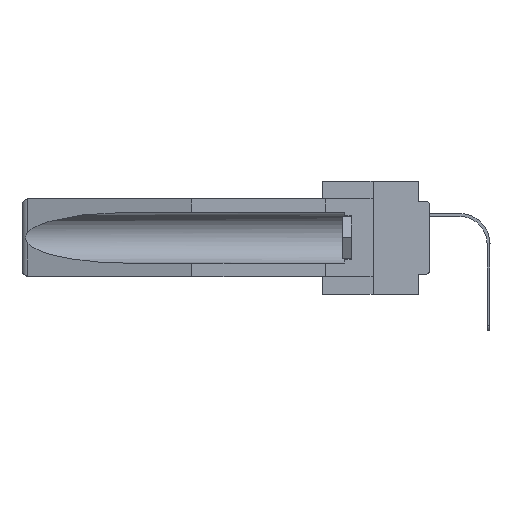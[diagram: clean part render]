
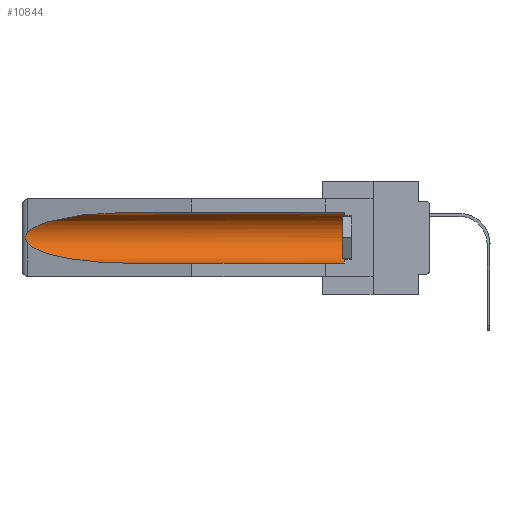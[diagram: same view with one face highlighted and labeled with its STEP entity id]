
A CAD part, left-side view. The second image highlights one B-rep face of the part: STEP entity #10844.
In plain terms, the highlighted cylindrical face has radius 2.857 mm (diameter 5.715 mm), a partial arc.
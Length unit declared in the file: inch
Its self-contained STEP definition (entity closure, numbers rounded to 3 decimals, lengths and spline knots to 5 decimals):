
#101 = CARTESIAN_POINT ( 'NONE',  ( 0.155, 1.07973, -0.059 ) ) ;
#251 = EDGE_CURVE ( 'NONE', #33269, #22558, #8034, .T. ) ;
#351 = ORIENTED_EDGE ( 'NONE', *, *, #16936, .T. ) ;
#2207 = CARTESIAN_POINT ( 'NONE',  ( 0.26537, 1.52718, -0.19328 ) ) ;
#2645 = FACE_OUTER_BOUND ( 'NONE', #35296, .T. ) ;
#2699 = CARTESIAN_POINT ( 'NONE',  ( 0.21114, 1.30732, -0.059 ) ) ;
#2713 = CARTESIAN_POINT ( 'NONE',  ( 0.26537, 1.52718, -0.14972 ) ) ;
#4264 = VERTEX_POINT ( 'NONE', #10974 ) ;
#4748 = CARTESIAN_POINT ( 'NONE',  ( 0.2675, 1.53308, -0.17534 ) ) ;
#4866 = DIRECTION ( 'NONE',  ( 0., 1., 0. ) ) ;
#5218 = CARTESIAN_POINT ( 'NONE',  ( 0.155, -0.30754, -0.1715 ) ) ;
#6916 =( BOUNDED_CURVE ( )  B_SPLINE_CURVE ( 3, ( #28275, #2699, #36361, #19280 ),
 .UNSPECIFIED., .F., .F. ) 
 B_SPLINE_CURVE_WITH_KNOTS ( ( 4, 4 ),
 ( 4.71239, 6.08839 ),
 .UNSPECIFIED. ) 
 CURVE ( )  GEOMETRIC_REPRESENTATION_ITEM ( )  RATIONAL_B_SPLINE_CURVE ( ( 1., 0.848, 0.848, 1. ) ) 
 REPRESENTATION_ITEM ( '' )  );
#7630 = CYLINDRICAL_SURFACE ( 'NONE', #23578, 0.1125 ) ;
#8034 =( BOUNDED_CURVE ( )  B_SPLINE_CURVE ( 3, ( #2207, #32602, #13428, #27257 ),
 .UNSPECIFIED., .F., .F. ) 
 B_SPLINE_CURVE_WITH_KNOTS ( ( 4, 4 ),
 ( 0.1948, 1.5708 ),
 .UNSPECIFIED. ) 
 CURVE ( )  GEOMETRIC_REPRESENTATION_ITEM ( )  RATIONAL_B_SPLINE_CURVE ( ( 1., 0.848, 0.848, 1. ) ) 
 REPRESENTATION_ITEM ( '' )  );
#10450 = CARTESIAN_POINT ( 'NONE',  ( 0.2675, 1.53308, -0.16763 ) ) ;
#10817 = CARTESIAN_POINT ( 'NONE',  ( 0.2673, 1.53269, -0.17917 ) ) ;
#10844 = ADVANCED_FACE ( 'NONE', ( #2645 ), #7630, .F. ) ;
#10974 = CARTESIAN_POINT ( 'NONE',  ( 0.26537, 1.52718, -0.14972 ) ) ;
#10988 = CARTESIAN_POINT ( 'NONE',  ( 0.2673, 1.5327, -0.16383 ) ) ;
#11410 = CARTESIAN_POINT ( 'NONE',  ( 0.155, -0.30754, -0.059 ) ) ;
#13428 = CARTESIAN_POINT ( 'NONE',  ( 0.21114, 1.30732, -0.284 ) ) ;
#15003 = ORIENTED_EDGE ( 'NONE', *, *, #26054, .T. ) ;
#16111 = DIRECTION ( 'NONE',  ( 0., 0., 1. ) ) ;
#16357 = CARTESIAN_POINT ( 'NONE',  ( 0.26655, 1.53094, -0.18657 ) ) ;
#16361 = ORIENTED_EDGE ( 'NONE', *, *, #30472, .T. ) ;
#16503 = CARTESIAN_POINT ( 'NONE',  ( 0.155, 0.126, -0.1715 ) ) ;
#16530 = VERTEX_POINT ( 'NONE', #23281 ) ;
#16885 = CARTESIAN_POINT ( 'NONE',  ( 0.155, 0.126, -0.284 ) ) ;
#16936 = EDGE_CURVE ( 'NONE', #16530, #33518, #25042, .T. ) ;
#19280 = CARTESIAN_POINT ( 'NONE',  ( 0.26537, 1.52718, -0.14972 ) ) ;
#20208 = VECTOR ( 'NONE', #27807, 39.37008 ) ;
#21665 = CARTESIAN_POINT ( 'NONE',  ( 0.26654, 1.53092, -0.15636 ) ) ;
#22036 = CARTESIAN_POINT ( 'NONE',  ( 0.26597, 1.5296, -0.19026 ) ) ;
#22558 = VERTEX_POINT ( 'NONE', #35323 ) ;
#22901 = EDGE_CURVE ( 'NONE', #34503, #22558, #34196, .T. ) ;
#23185 = EDGE_CURVE ( 'NONE', #33518, #4264, #6916, .T. ) ;
#23281 = CARTESIAN_POINT ( 'NONE',  ( 0.155, 0.126, -0.059 ) ) ;
#23578 = AXIS2_PLACEMENT_3D ( 'NONE', #5218, #4866, #16111 ) ;
#24031 = CARTESIAN_POINT ( 'NONE',  ( 0.26537, 1.52718, -0.19328 ) ) ;
#24969 = ORIENTED_EDGE ( 'NONE', *, *, #251, .T. ) ;
#25042 = LINE ( 'NONE', #11410, #20208 ) ;
#25130 = DIRECTION ( 'NONE',  ( 0., 0., 1. ) ) ;
#26054 = EDGE_CURVE ( 'NONE', #34503, #16530, #35361, .T. ) ;
#26657 = CARTESIAN_POINT ( 'NONE',  ( 0.155, -0.30754, -0.284 ) ) ;
#27257 = CARTESIAN_POINT ( 'NONE',  ( 0.155, 1.07973, -0.284 ) ) ;
#27548 = B_SPLINE_CURVE_WITH_KNOTS ( 'NONE', 3,
 ( #2713, #30499, #21665, #10988, #10450, #4748, #10817, #16357, #22036, #32912 ),
 .UNSPECIFIED., .F., .F.,
 ( 4, 2, 2, 2, 4 ),
 ( 0., 0.00029, 0.00058, 0.00087, 0.00117 ),
 .UNSPECIFIED. ) ;
#27807 = DIRECTION ( 'NONE',  ( 0., 1., 0. ) ) ;
#28275 = CARTESIAN_POINT ( 'NONE',  ( 0.155, 1.07973, -0.059 ) ) ;
#29250 = DIRECTION ( 'NONE',  ( 0., 1., 0. ) ) ;
#30117 = ORIENTED_EDGE ( 'NONE', *, *, #22901, .F. ) ;
#30472 = EDGE_CURVE ( 'NONE', #4264, #33269, #27548, .T. ) ;
#30499 = CARTESIAN_POINT ( 'NONE',  ( 0.26597, 1.52961, -0.15275 ) ) ;
#31248 = AXIS2_PLACEMENT_3D ( 'NONE', #16503, #36183, #25130 ) ;
#31999 = ORIENTED_EDGE ( 'NONE', *, *, #23185, .T. ) ;
#32602 = CARTESIAN_POINT ( 'NONE',  ( 0.25451, 1.48313, -0.24835 ) ) ;
#32912 = CARTESIAN_POINT ( 'NONE',  ( 0.26537, 1.52718, -0.19328 ) ) ;
#33269 = VERTEX_POINT ( 'NONE', #24031 ) ;
#33518 = VERTEX_POINT ( 'NONE', #101 ) ;
#34080 = VECTOR ( 'NONE', #29250, 39.37008 ) ;
#34196 = LINE ( 'NONE', #26657, #34080 ) ;
#34503 = VERTEX_POINT ( 'NONE', #16885 ) ;
#35296 = EDGE_LOOP ( 'NONE', ( #31999, #16361, #24969, #30117, #15003, #351 ) ) ;
#35323 = CARTESIAN_POINT ( 'NONE',  ( 0.155, 1.07973, -0.284 ) ) ;
#35361 = CIRCLE ( 'NONE', #31248, 0.1125 ) ;
#36183 = DIRECTION ( 'NONE',  ( 0., -1., 0. ) ) ;
#36361 = CARTESIAN_POINT ( 'NONE',  ( 0.25451, 1.48313, -0.09465 ) ) ;
